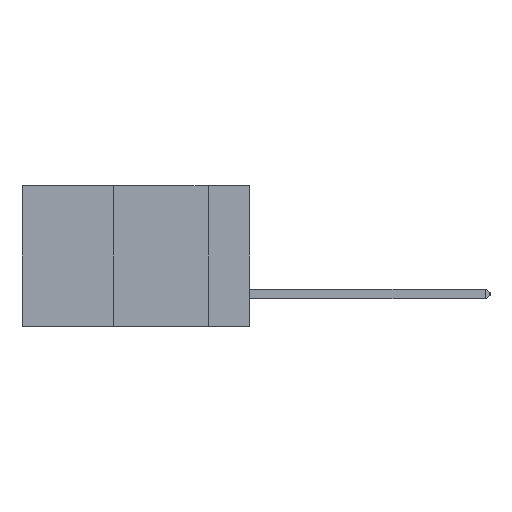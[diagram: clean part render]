
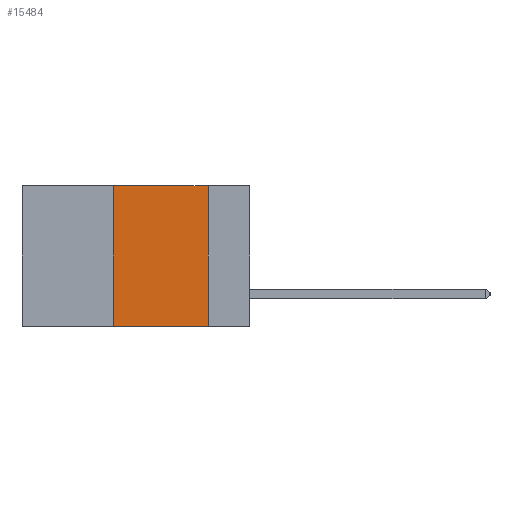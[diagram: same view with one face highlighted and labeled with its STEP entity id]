
A CAD part, left-side view. The second image highlights one B-rep face of the part: STEP entity #15484.
In plain terms, the highlighted planar face has unit normal (-1, 0, 0).
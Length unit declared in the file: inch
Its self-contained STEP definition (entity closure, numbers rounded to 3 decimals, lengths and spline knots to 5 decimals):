
#658 = FACE_OUTER_BOUND ( 'NONE', #10098, .T. ) ;
#811 = VECTOR ( 'NONE', #24880, 39.37008 ) ;
#912 = ORIENTED_EDGE ( 'NONE', *, *, #12672, .T. ) ;
#1356 = CARTESIAN_POINT ( 'NONE',  ( 0., 0.6, -0.37 ) ) ;
#5677 = DIRECTION ( 'NONE',  ( 1., 0., 0. ) ) ;
#6750 = LINE ( 'NONE', #22957, #811 ) ;
#6763 = VERTEX_POINT ( 'NONE', #7767 ) ;
#6777 = LINE ( 'NONE', #7392, #10776 ) ;
#6852 = AXIS2_PLACEMENT_3D ( 'NONE', #7540, #5677, #19495 ) ;
#6896 = VERTEX_POINT ( 'NONE', #16156 ) ;
#7392 = CARTESIAN_POINT ( 'NONE',  ( 0., 0.36, 0. ) ) ;
#7540 = CARTESIAN_POINT ( 'NONE',  ( 0., 0.6, 0. ) ) ;
#7767 = CARTESIAN_POINT ( 'NONE',  ( 0., 0.11, 0. ) ) ;
#9487 = VERTEX_POINT ( 'NONE', #16565 ) ;
#10098 = EDGE_LOOP ( 'NONE', ( #13955, #21036, #16758, #912 ) ) ;
#10776 = VECTOR ( 'NONE', #17350, 39.37008 ) ;
#11406 = CARTESIAN_POINT ( 'NONE',  ( 0., 0.36, -0.37 ) ) ;
#11705 = CARTESIAN_POINT ( 'NONE',  ( 0., 0.11, 0. ) ) ;
#12090 = VERTEX_POINT ( 'NONE', #11406 ) ;
#12672 = EDGE_CURVE ( 'NONE', #12090, #6896, #24434, .T. ) ;
#13711 = DIRECTION ( 'NONE',  ( 0., 0., -1. ) ) ;
#13955 = ORIENTED_EDGE ( 'NONE', *, *, #21942, .F. ) ;
#15281 = VECTOR ( 'NONE', #13711, 39.37008 ) ;
#15484 = ADVANCED_FACE ( 'NONE', ( #658 ), #17501, .F. ) ;
#16156 = CARTESIAN_POINT ( 'NONE',  ( 0., 0.11, -0.37 ) ) ;
#16514 = LINE ( 'NONE', #11705, #15281 ) ;
#16565 = CARTESIAN_POINT ( 'NONE',  ( 0., 0.36, 0. ) ) ;
#16758 = ORIENTED_EDGE ( 'NONE', *, *, #17834, .F. ) ;
#17195 = DIRECTION ( 'NONE',  ( 0., -1., 0. ) ) ;
#17350 = DIRECTION ( 'NONE',  ( 0., 0., 1. ) ) ;
#17501 = PLANE ( 'NONE',  #6852 ) ;
#17834 = EDGE_CURVE ( 'NONE', #12090, #9487, #6777, .T. ) ;
#18298 = EDGE_CURVE ( 'NONE', #9487, #6763, #6750, .T. ) ;
#18691 = VECTOR ( 'NONE', #17195, 39.37008 ) ;
#19495 = DIRECTION ( 'NONE',  ( 0., 0., -1. ) ) ;
#21036 = ORIENTED_EDGE ( 'NONE', *, *, #18298, .F. ) ;
#21942 = EDGE_CURVE ( 'NONE', #6763, #6896, #16514, .T. ) ;
#22957 = CARTESIAN_POINT ( 'NONE',  ( 0., 0.6, 0. ) ) ;
#24434 = LINE ( 'NONE', #1356, #18691 ) ;
#24880 = DIRECTION ( 'NONE',  ( 0., -1., 0. ) ) ;
